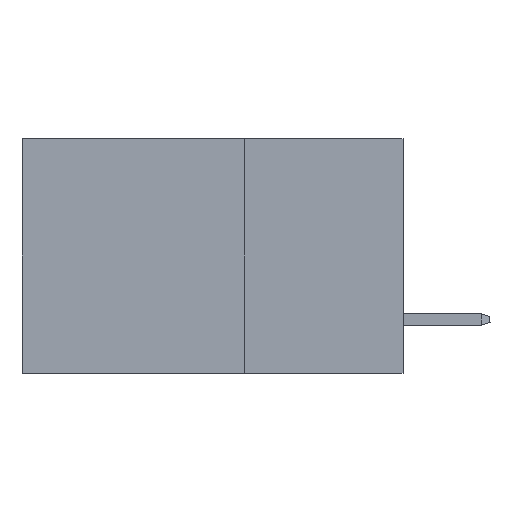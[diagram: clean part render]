
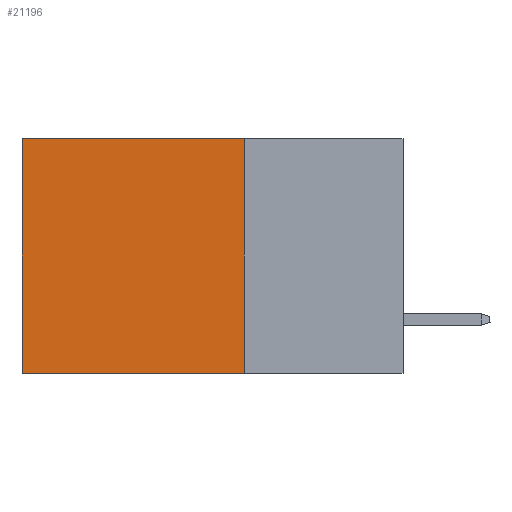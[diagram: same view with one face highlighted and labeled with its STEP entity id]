
A CAD part, left-side view. The second image highlights one B-rep face of the part: STEP entity #21196.
In plain terms, the highlighted planar face has unit normal (-1, 0, 0).
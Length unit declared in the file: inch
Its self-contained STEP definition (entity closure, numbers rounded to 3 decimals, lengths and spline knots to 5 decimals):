
#283 = CARTESIAN_POINT ( 'NONE',  ( 0.2875, 0.25, 0. ) ) ;
#981 = PLANE ( 'NONE',  #12637 ) ;
#1018 = LINE ( 'NONE', #2839, #22698 ) ;
#1805 = EDGE_CURVE ( 'NONE', #16182, #15676, #6915, .T. ) ;
#1978 = VERTEX_POINT ( 'NONE', #22021 ) ;
#2573 = VERTEX_POINT ( 'NONE', #283 ) ;
#2839 = CARTESIAN_POINT ( 'NONE',  ( 0.2875, 0.25, -0.37 ) ) ;
#3401 = ORIENTED_EDGE ( 'NONE', *, *, #13474, .F. ) ;
#3613 = DIRECTION ( 'NONE',  ( 0., 0., -1. ) ) ;
#4825 = EDGE_CURVE ( 'NONE', #2573, #16182, #14196, .T. ) ;
#5335 = DIRECTION ( 'NONE',  ( 0., 1., 0. ) ) ;
#6645 = VECTOR ( 'NONE', #3613, 39.37008 ) ;
#6883 = ORIENTED_EDGE ( 'NONE', *, *, #15565, .F. ) ;
#6915 = LINE ( 'NONE', #19565, #6645 ) ;
#8727 = CARTESIAN_POINT ( 'NONE',  ( 0.2875, 0.25, 0. ) ) ;
#9052 = VECTOR ( 'NONE', #5335, 39.37008 ) ;
#9964 = DIRECTION ( 'NONE',  ( 0., 1., 0. ) ) ;
#10132 = ORIENTED_EDGE ( 'NONE', *, *, #1805, .T. ) ;
#11484 = VECTOR ( 'NONE', #15824, 39.37008 ) ;
#12232 = CARTESIAN_POINT ( 'NONE',  ( 0.2875, 0.25, 0. ) ) ;
#12637 = AXIS2_PLACEMENT_3D ( 'NONE', #22261, #22385, #13441 ) ;
#13441 = DIRECTION ( 'NONE',  ( 0., 0., -1. ) ) ;
#13474 = EDGE_CURVE ( 'NONE', #2573, #1978, #13958, .T. ) ;
#13780 = FACE_OUTER_BOUND ( 'NONE', #17920, .T. ) ;
#13958 = LINE ( 'NONE', #8727, #11484 ) ;
#14196 = LINE ( 'NONE', #12232, #9052 ) ;
#14487 = ORIENTED_EDGE ( 'NONE', *, *, #4825, .T. ) ;
#15565 = EDGE_CURVE ( 'NONE', #1978, #15676, #1018, .T. ) ;
#15676 = VERTEX_POINT ( 'NONE', #17216 ) ;
#15824 = DIRECTION ( 'NONE',  ( 0., 0., -1. ) ) ;
#16182 = VERTEX_POINT ( 'NONE', #18742 ) ;
#17216 = CARTESIAN_POINT ( 'NONE',  ( 0.2875, 0.6, -0.37 ) ) ;
#17920 = EDGE_LOOP ( 'NONE', ( #10132, #6883, #3401, #14487 ) ) ;
#18742 = CARTESIAN_POINT ( 'NONE',  ( 0.2875, 0.6, 0. ) ) ;
#19565 = CARTESIAN_POINT ( 'NONE',  ( 0.2875, 0.6, 0. ) ) ;
#21196 = ADVANCED_FACE ( 'NONE', ( #13780 ), #981, .F. ) ;
#22021 = CARTESIAN_POINT ( 'NONE',  ( 0.2875, 0.25, -0.37 ) ) ;
#22261 = CARTESIAN_POINT ( 'NONE',  ( 0.2875, 0.25, 0. ) ) ;
#22385 = DIRECTION ( 'NONE',  ( 1., 0., 0. ) ) ;
#22698 = VECTOR ( 'NONE', #9964, 39.37008 ) ;
